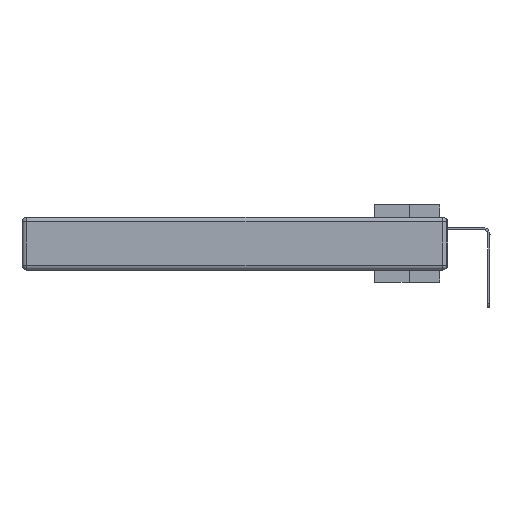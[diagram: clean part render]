
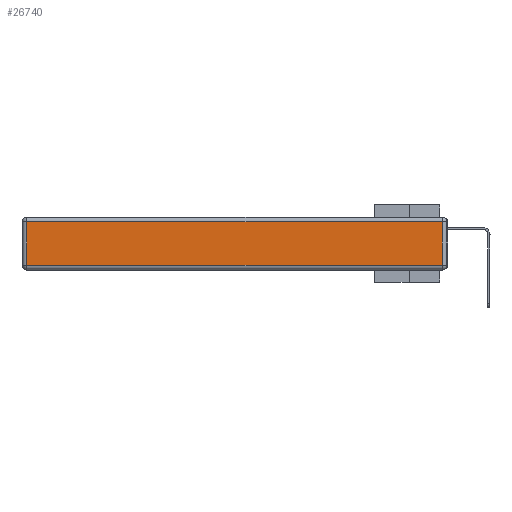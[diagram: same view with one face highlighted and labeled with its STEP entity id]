
A CAD part, left-side view. The second image highlights one B-rep face of the part: STEP entity #26740.
In plain terms, the highlighted planar face has unit normal (-1, 0, 0).
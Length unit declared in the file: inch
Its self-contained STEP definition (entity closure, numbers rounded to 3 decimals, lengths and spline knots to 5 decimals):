
#21 = ORIENTED_EDGE ( 'NONE', *, *, #21485, .T. ) ;
#1690 = VECTOR ( 'NONE', #3044, 39.37008 ) ;
#2431 = VECTOR ( 'NONE', #23387, 39.37008 ) ;
#3044 = DIRECTION ( 'NONE',  ( 0., 1., 0. ) ) ;
#4438 = ORIENTED_EDGE ( 'NONE', *, *, #15602, .T. ) ;
#5261 = CARTESIAN_POINT ( 'NONE',  ( 0., 2.72, -0.343 ) ) ;
#6328 = PLANE ( 'NONE',  #17424 ) ;
#6845 = ORIENTED_EDGE ( 'NONE', *, *, #23010, .T. ) ;
#7618 = CARTESIAN_POINT ( 'NONE',  ( 0., 2.72, -0.313 ) ) ;
#8428 = CARTESIAN_POINT ( 'NONE',  ( 0., 0.03, -0.03 ) ) ;
#9730 = DIRECTION ( 'NONE',  ( 0., 0., 1. ) ) ;
#10093 = VERTEX_POINT ( 'NONE', #25241 ) ;
#10217 = CARTESIAN_POINT ( 'NONE',  ( 0., 2.72, -0.03 ) ) ;
#10379 = DIRECTION ( 'NONE',  ( -1., 0., 0. ) ) ;
#14235 = CARTESIAN_POINT ( 'NONE',  ( 0., 0.03, -0.343 ) ) ;
#14583 = VERTEX_POINT ( 'NONE', #8428 ) ;
#15041 = CARTESIAN_POINT ( 'NONE',  ( 0., 0., -0.313 ) ) ;
#15602 = EDGE_CURVE ( 'NONE', #15776, #16128, #27228, .T. ) ;
#15776 = VERTEX_POINT ( 'NONE', #10217 ) ;
#15867 = CARTESIAN_POINT ( 'NONE',  ( 0., 2.75, -0.03 ) ) ;
#16044 = EDGE_CURVE ( 'NONE', #14583, #15776, #22626, .T. ) ;
#16128 = VERTEX_POINT ( 'NONE', #7618 ) ;
#17424 = AXIS2_PLACEMENT_3D ( 'NONE', #21991, #10379, #28465 ) ;
#17608 = ORIENTED_EDGE ( 'NONE', *, *, #16044, .T. ) ;
#18141 = VECTOR ( 'NONE', #21770, 39.37008 ) ;
#21485 = EDGE_CURVE ( 'NONE', #10093, #14583, #22155, .T. ) ;
#21770 = DIRECTION ( 'NONE',  ( 0., -1., 0. ) ) ;
#21991 = CARTESIAN_POINT ( 'NONE',  ( 0., 0., -0.343 ) ) ;
#22033 = FACE_OUTER_BOUND ( 'NONE', #25999, .T. ) ;
#22155 = LINE ( 'NONE', #14235, #27411 ) ;
#22626 = LINE ( 'NONE', #15867, #1690 ) ;
#23010 = EDGE_CURVE ( 'NONE', #16128, #10093, #27669, .T. ) ;
#23387 = DIRECTION ( 'NONE',  ( 0., 0., -1. ) ) ;
#25241 = CARTESIAN_POINT ( 'NONE',  ( 0., 0.03, -0.313 ) ) ;
#25999 = EDGE_LOOP ( 'NONE', ( #6845, #21, #17608, #4438 ) ) ;
#26740 = ADVANCED_FACE ( 'NONE', ( #22033 ), #6328, .T. ) ;
#27228 = LINE ( 'NONE', #5261, #2431 ) ;
#27411 = VECTOR ( 'NONE', #9730, 39.37008 ) ;
#27669 = LINE ( 'NONE', #15041, #18141 ) ;
#28465 = DIRECTION ( 'NONE',  ( 0., 0., 1. ) ) ;
